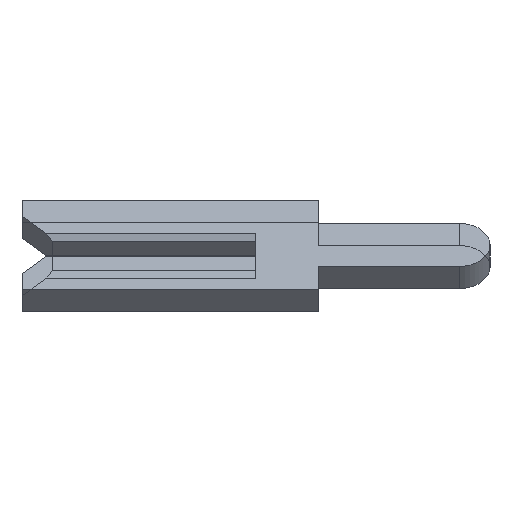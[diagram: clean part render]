
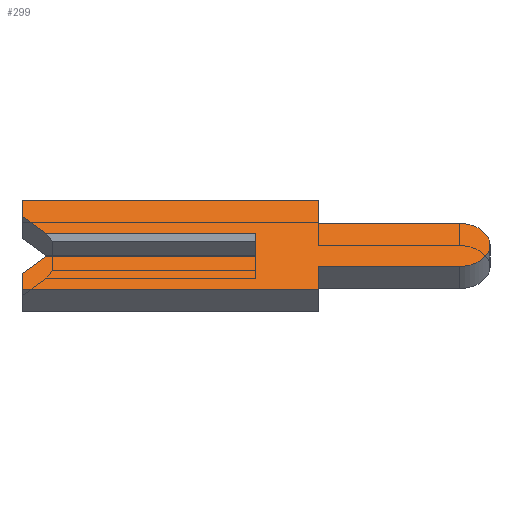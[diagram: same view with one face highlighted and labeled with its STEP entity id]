
A CAD part, left-side view. The second image highlights one B-rep face of the part: STEP entity #299.
In plain terms, the highlighted face is planar.
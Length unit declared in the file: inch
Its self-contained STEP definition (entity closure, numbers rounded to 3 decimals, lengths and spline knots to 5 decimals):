
#40 = CARTESIAN_POINT ( 'NONE',  ( -0.01, 0.15, 0.04 ) ) ;
#42 = VERTEX_POINT ( 'NONE', #982 ) ;
#60 = CARTESIAN_POINT ( 'NONE',  ( -0.01, -0.1305, -0.01 ) ) ;
#78 = DIRECTION ( 'NONE',  ( 0., 0., 1. ) ) ;
#80 = VECTOR ( 'NONE', #1465, 39.37008 ) ;
#156 = VECTOR ( 'NONE', #1590, 39.37008 ) ;
#166 = ORIENTED_EDGE ( 'NONE', *, *, #2367, .F. ) ;
#190 = LINE ( 'NONE', #60, #2691 ) ;
#228 = VERTEX_POINT ( 'NONE', #1489 ) ;
#246 = VECTOR ( 'NONE', #1468, 39.37008 ) ;
#247 = ORIENTED_EDGE ( 'NONE', *, *, #2757, .F. ) ;
#299 = ADVANCED_FACE ( 'NONE', ( #2281 ), #501, .F. ) ;
#305 = EDGE_CURVE ( 'NONE', #1476, #713, #2324, .T. ) ;
#309 = LINE ( 'NONE', #759, #2815 ) ;
#464 = VECTOR ( 'NONE', #1319, 39.37008 ) ;
#474 = DIRECTION ( 'NONE',  ( 0., 0., 1. ) ) ;
#490 = CARTESIAN_POINT ( 'NONE',  ( -0.01, -0.04, 0.0195 ) ) ;
#501 = PLANE ( 'NONE',  #773 ) ;
#536 = VECTOR ( 'NONE', #78, 39.37008 ) ;
#537 = DIRECTION ( 'NONE',  ( 0., 1., 0. ) ) ;
#560 = DIRECTION ( 'NONE',  ( 0., -1., 0. ) ) ;
#591 = DIRECTION ( 'NONE',  ( 1., 0., 0. ) ) ;
#595 = ORIENTED_EDGE ( 'NONE', *, *, #1114, .F. ) ;
#664 = CARTESIAN_POINT ( 'NONE',  ( -0.01, -0.04, 0.0195 ) ) ;
#698 = CARTESIAN_POINT ( 'NONE',  ( -0.01, -0.04, -0.04 ) ) ;
#713 = VERTEX_POINT ( 'NONE', #1544 ) ;
#737 = CARTESIAN_POINT ( 'NONE',  ( -0.01, 0.15, 0.04 ) ) ;
#743 = ORIENTED_EDGE ( 'NONE', *, *, #957, .F. ) ;
#759 = CARTESIAN_POINT ( 'NONE',  ( -0.01, 0.15, -0.026 ) ) ;
#773 = AXIS2_PLACEMENT_3D ( 'NONE', #1984, #591, #1715 ) ;
#805 = CIRCLE ( 'NONE', #3003, 0.0195 ) ;
#859 = LINE ( 'NONE', #1519, #2536 ) ;
#915 = CARTESIAN_POINT ( 'NONE',  ( -0.01, 0.1305, 0.0065 ) ) ;
#932 = EDGE_CURVE ( 'NONE', #1082, #1696, #859, .T. ) ;
#957 = EDGE_CURVE ( 'NONE', #42, #1093, #3008, .T. ) ;
#982 = CARTESIAN_POINT ( 'NONE',  ( -0.01, -0.1305, -0.0195 ) ) ;
#1014 = ORIENTED_EDGE ( 'NONE', *, *, #2647, .F. ) ;
#1054 = CARTESIAN_POINT ( 'NONE',  ( -0.01, -0.04, -0.0195 ) ) ;
#1057 = EDGE_CURVE ( 'NONE', #1512, #2887, #1229, .T. ) ;
#1071 = ORIENTED_EDGE ( 'NONE', *, *, #2515, .F. ) ;
#1082 = VERTEX_POINT ( 'NONE', #2804 ) ;
#1093 = VERTEX_POINT ( 'NONE', #1259 ) ;
#1094 = CARTESIAN_POINT ( 'NONE',  ( -0.01, 0.15, 0.026 ) ) ;
#1114 = EDGE_CURVE ( 'NONE', #2200, #1476, #2353, .T. ) ;
#1179 = LINE ( 'NONE', #40, #2111 ) ;
#1185 = LINE ( 'NONE', #3102, #156 ) ;
#1229 = LINE ( 'NONE', #2782, #536 ) ;
#1259 = CARTESIAN_POINT ( 'NONE',  ( -0.01, -0.04, -0.0195 ) ) ;
#1280 = EDGE_LOOP ( 'NONE', ( #2180, #1922, #166, #2867, #247, #1014, #2545, #743, #1071, #2080, #595, #2084, #3046, #2715 ) ) ;
#1282 = EDGE_CURVE ( 'NONE', #228, #1354, #1185, .T. ) ;
#1319 = DIRECTION ( 'NONE',  ( 0., 0.707, 0.707 ) ) ;
#1354 = VERTEX_POINT ( 'NONE', #1581 ) ;
#1387 = EDGE_CURVE ( 'NONE', #1082, #1512, #1706, .T. ) ;
#1413 = LINE ( 'NONE', #1725, #2777 ) ;
#1416 = CARTESIAN_POINT ( 'NONE',  ( -0.01, -0.04, 0.04 ) ) ;
#1465 = DIRECTION ( 'NONE',  ( 0., 1., 0. ) ) ;
#1468 = DIRECTION ( 'NONE',  ( 0., -1., 0. ) ) ;
#1476 = VERTEX_POINT ( 'NONE', #664 ) ;
#1489 = CARTESIAN_POINT ( 'NONE',  ( -0.01, 0.15, -0.026 ) ) ;
#1507 = DIRECTION ( 'NONE',  ( 0., 0., -1. ) ) ;
#1512 = VERTEX_POINT ( 'NONE', #1094 ) ;
#1519 = CARTESIAN_POINT ( 'NONE',  ( -0.01, 0.15, 0.01 ) ) ;
#1544 = CARTESIAN_POINT ( 'NONE',  ( -0.01, -0.1305, 0.0195 ) ) ;
#1581 = CARTESIAN_POINT ( 'NONE',  ( -0.01, 0.134, -0.01 ) ) ;
#1590 = DIRECTION ( 'NONE',  ( 0., -0.707, 0.707 ) ) ;
#1696 = VERTEX_POINT ( 'NONE', #3093 ) ;
#1706 = LINE ( 'NONE', #915, #464 ) ;
#1715 = DIRECTION ( 'NONE',  ( 0., 0., -1. ) ) ;
#1725 = CARTESIAN_POINT ( 'NONE',  ( -0.01, -0.04, -0.04 ) ) ;
#1772 = CARTESIAN_POINT ( 'NONE',  ( -0.01, 0., -0.01 ) ) ;
#1922 = ORIENTED_EDGE ( 'NONE', *, *, #2248, .F. ) ;
#1981 = CARTESIAN_POINT ( 'NONE',  ( -0.01, 0.15, -0.04 ) ) ;
#1984 = CARTESIAN_POINT ( 'NONE',  ( -0.01, -0.1305, 0. ) ) ;
#2028 = CARTESIAN_POINT ( 'NONE',  ( -0.01, -0.1305, 0. ) ) ;
#2037 = DIRECTION ( 'NONE',  ( 0., -1., 0. ) ) ;
#2063 = VERTEX_POINT ( 'NONE', #698 ) ;
#2080 = ORIENTED_EDGE ( 'NONE', *, *, #305, .F. ) ;
#2084 = ORIENTED_EDGE ( 'NONE', *, *, #2477, .F. ) ;
#2111 = VECTOR ( 'NONE', #2275, 39.37008 ) ;
#2140 = VERTEX_POINT ( 'NONE', #2709 ) ;
#2180 = ORIENTED_EDGE ( 'NONE', *, *, #932, .T. ) ;
#2200 = VERTEX_POINT ( 'NONE', #1416 ) ;
#2222 = LINE ( 'NONE', #1981, #80 ) ;
#2248 = EDGE_CURVE ( 'NONE', #2899, #1696, #2734, .T. ) ;
#2275 = DIRECTION ( 'NONE',  ( 0., -1., 0. ) ) ;
#2281 = FACE_OUTER_BOUND ( 'NONE', #1280, .T. ) ;
#2324 = LINE ( 'NONE', #490, #246 ) ;
#2336 = CARTESIAN_POINT ( 'NONE',  ( -0.01, -0.04, 0.04 ) ) ;
#2353 = LINE ( 'NONE', #2336, #2742 ) ;
#2367 = EDGE_CURVE ( 'NONE', #1354, #2899, #190, .T. ) ;
#2423 = VECTOR ( 'NONE', #537, 39.37008 ) ;
#2477 = EDGE_CURVE ( 'NONE', #2887, #2200, #1179, .T. ) ;
#2515 = EDGE_CURVE ( 'NONE', #713, #42, #805, .T. ) ;
#2536 = VECTOR ( 'NONE', #2037, 39.37008 ) ;
#2545 = ORIENTED_EDGE ( 'NONE', *, *, #2918, .F. ) ;
#2647 = EDGE_CURVE ( 'NONE', #2063, #2140, #2222, .T. ) ;
#2691 = VECTOR ( 'NONE', #560, 39.37008 ) ;
#2709 = CARTESIAN_POINT ( 'NONE',  ( -0.01, 0.15, -0.04 ) ) ;
#2715 = ORIENTED_EDGE ( 'NONE', *, *, #1387, .F. ) ;
#2734 = LINE ( 'NONE', #2924, #3120 ) ;
#2742 = VECTOR ( 'NONE', #3044, 39.37008 ) ;
#2757 = EDGE_CURVE ( 'NONE', #2140, #228, #309, .T. ) ;
#2761 = DIRECTION ( 'NONE',  ( 1., 0., 0. ) ) ;
#2777 = VECTOR ( 'NONE', #1507, 39.37008 ) ;
#2781 = DIRECTION ( 'NONE',  ( 0., 0., -1. ) ) ;
#2782 = CARTESIAN_POINT ( 'NONE',  ( -0.01, 0.15, 0.026 ) ) ;
#2804 = CARTESIAN_POINT ( 'NONE',  ( -0.01, 0.134, 0.01 ) ) ;
#2815 = VECTOR ( 'NONE', #3015, 39.37008 ) ;
#2867 = ORIENTED_EDGE ( 'NONE', *, *, #1282, .F. ) ;
#2887 = VERTEX_POINT ( 'NONE', #737 ) ;
#2899 = VERTEX_POINT ( 'NONE', #1772 ) ;
#2918 = EDGE_CURVE ( 'NONE', #1093, #2063, #1413, .T. ) ;
#2924 = CARTESIAN_POINT ( 'NONE',  ( -0.01, 0., 0.0065 ) ) ;
#3003 = AXIS2_PLACEMENT_3D ( 'NONE', #2028, #2761, #2781 ) ;
#3008 = LINE ( 'NONE', #1054, #2423 ) ;
#3015 = DIRECTION ( 'NONE',  ( 0., 0., 1. ) ) ;
#3044 = DIRECTION ( 'NONE',  ( 0., 0., -1. ) ) ;
#3046 = ORIENTED_EDGE ( 'NONE', *, *, #1057, .F. ) ;
#3093 = CARTESIAN_POINT ( 'NONE',  ( -0.01, 0., 0.01 ) ) ;
#3102 = CARTESIAN_POINT ( 'NONE',  ( -0.01, 0.1305, -0.0065 ) ) ;
#3120 = VECTOR ( 'NONE', #474, 39.37008 ) ;
